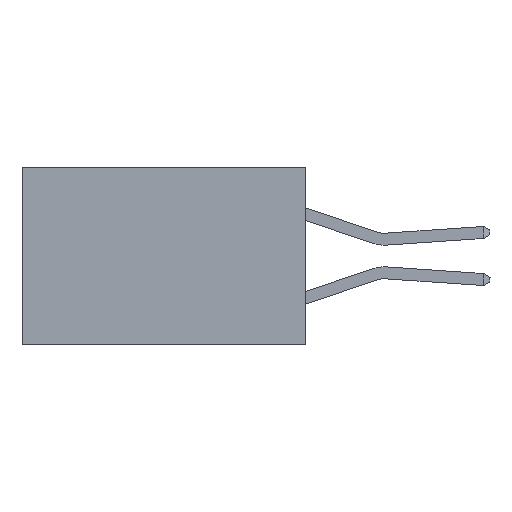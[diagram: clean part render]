
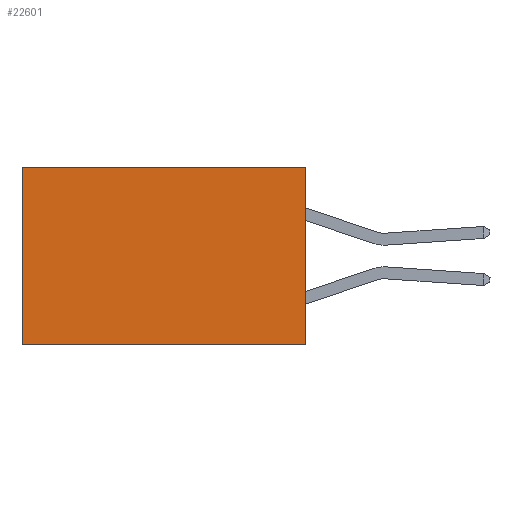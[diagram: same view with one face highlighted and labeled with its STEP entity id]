
A CAD part, left-side view. The second image highlights one B-rep face of the part: STEP entity #22601.
In plain terms, the highlighted planar face has unit normal (-1, 0, 0).
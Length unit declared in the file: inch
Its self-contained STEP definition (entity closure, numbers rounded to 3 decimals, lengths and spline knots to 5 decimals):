
#812 = ORIENTED_EDGE ( 'NONE', *, *, #22445, .F. ) ;
#2195 = LINE ( 'NONE', #17917, #21876 ) ;
#2394 = CARTESIAN_POINT ( 'NONE',  ( 0.277, 0., -0.37 ) ) ;
#2981 = CARTESIAN_POINT ( 'NONE',  ( 0.277, 0.59, 0. ) ) ;
#3147 = CARTESIAN_POINT ( 'NONE',  ( 0.277, 0., 0. ) ) ;
#3154 = FACE_OUTER_BOUND ( 'NONE', #20885, .T. ) ;
#3641 = VERTEX_POINT ( 'NONE', #20689 ) ;
#5088 = DIRECTION ( 'NONE',  ( 0., 1., 0. ) ) ;
#5580 = VERTEX_POINT ( 'NONE', #2981 ) ;
#5802 = DIRECTION ( 'NONE',  ( 0., 0., -1. ) ) ;
#7026 = EDGE_CURVE ( 'NONE', #5580, #15099, #22994, .T. ) ;
#7757 = CARTESIAN_POINT ( 'NONE',  ( 0.277, 0., -0.37 ) ) ;
#8225 = PLANE ( 'NONE',  #9064 ) ;
#8307 = ORIENTED_EDGE ( 'NONE', *, *, #14291, .T. ) ;
#8472 = DIRECTION ( 'NONE',  ( 0., 1., 0. ) ) ;
#8482 = VECTOR ( 'NONE', #10524, 39.37008 ) ;
#9064 = AXIS2_PLACEMENT_3D ( 'NONE', #2394, #10130, #23381 ) ;
#10130 = DIRECTION ( 'NONE',  ( 1., 0., 0. ) ) ;
#10325 = VECTOR ( 'NONE', #5088, 39.37008 ) ;
#10524 = DIRECTION ( 'NONE',  ( 0., 0., -1. ) ) ;
#11443 = VERTEX_POINT ( 'NONE', #13480 ) ;
#12107 = ORIENTED_EDGE ( 'NONE', *, *, #7026, .T. ) ;
#13480 = CARTESIAN_POINT ( 'NONE',  ( 0.277, 0., 0. ) ) ;
#14291 = EDGE_CURVE ( 'NONE', #11443, #5580, #20422, .T. ) ;
#15099 = VERTEX_POINT ( 'NONE', #18057 ) ;
#15430 = ORIENTED_EDGE ( 'NONE', *, *, #23297, .F. ) ;
#17242 = VECTOR ( 'NONE', #5802, 39.37008 ) ;
#17917 = CARTESIAN_POINT ( 'NONE',  ( 0.277, 0., -0.37 ) ) ;
#18057 = CARTESIAN_POINT ( 'NONE',  ( 0.277, 0.59, -0.37 ) ) ;
#20422 = LINE ( 'NONE', #3147, #10325 ) ;
#20689 = CARTESIAN_POINT ( 'NONE',  ( 0.277, 0., -0.37 ) ) ;
#20885 = EDGE_LOOP ( 'NONE', ( #12107, #15430, #812, #8307 ) ) ;
#21876 = VECTOR ( 'NONE', #8472, 39.37008 ) ;
#22189 = CARTESIAN_POINT ( 'NONE',  ( 0.277, 0.59, -0.37 ) ) ;
#22445 = EDGE_CURVE ( 'NONE', #11443, #3641, #24109, .T. ) ;
#22601 = ADVANCED_FACE ( 'NONE', ( #3154 ), #8225, .F. ) ;
#22994 = LINE ( 'NONE', #22189, #8482 ) ;
#23297 = EDGE_CURVE ( 'NONE', #3641, #15099, #2195, .T. ) ;
#23381 = DIRECTION ( 'NONE',  ( 0., 0., -1. ) ) ;
#24109 = LINE ( 'NONE', #7757, #17242 ) ;
